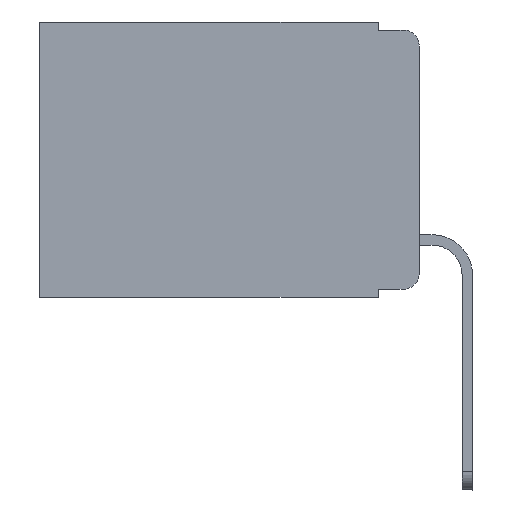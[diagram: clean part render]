
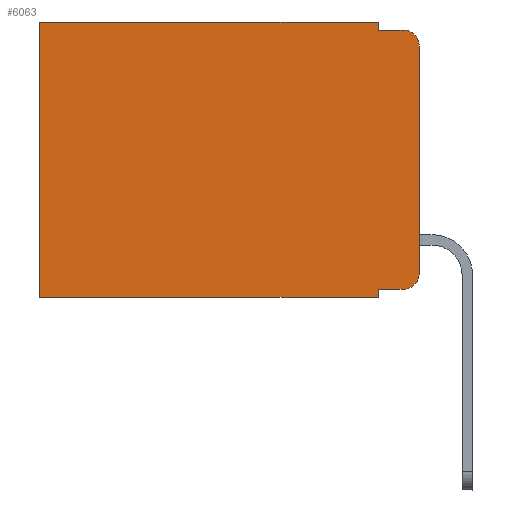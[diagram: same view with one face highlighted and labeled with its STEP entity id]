
A CAD part, left-side view. The second image highlights one B-rep face of the part: STEP entity #6063.
In plain terms, the highlighted planar face has unit normal (-1, 0, 0).
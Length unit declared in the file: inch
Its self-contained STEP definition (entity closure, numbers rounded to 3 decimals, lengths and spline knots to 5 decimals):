
#758 = CARTESIAN_POINT ( 'NONE',  ( 0.298, 0.473, -0.343 ) ) ;
#1137 = CARTESIAN_POINT ( 'NONE',  ( 0.298, 0., -0.03 ) ) ;
#1719 = VECTOR ( 'NONE', #22870, 39.37008 ) ;
#1736 = VERTEX_POINT ( 'NONE', #13730 ) ;
#1997 = CARTESIAN_POINT ( 'NONE',  ( 0.298, 0.02, -0.333 ) ) ;
#2095 = VERTEX_POINT ( 'NONE', #14075 ) ;
#2382 = VERTEX_POINT ( 'NONE', #1997 ) ;
#2701 = VECTOR ( 'NONE', #21764, 39.37008 ) ;
#2813 = VECTOR ( 'NONE', #3290, 39.37008 ) ;
#3217 = FACE_OUTER_BOUND ( 'NONE', #20248, .T. ) ;
#3290 = DIRECTION ( 'NONE',  ( 0., -1., 0. ) ) ;
#3627 = EDGE_CURVE ( 'NONE', #8540, #12872, #12313, .T. ) ;
#3735 = ORIENTED_EDGE ( 'NONE', *, *, #16666, .F. ) ;
#4019 = ORIENTED_EDGE ( 'NONE', *, *, #6465, .T. ) ;
#4311 = CARTESIAN_POINT ( 'NONE',  ( 0.298, 0.473, 0. ) ) ;
#5211 = CARTESIAN_POINT ( 'NONE',  ( 0.298, 0.051, 0. ) ) ;
#5522 = DIRECTION ( 'NONE',  ( -1., 0., 0. ) ) ;
#5570 = VECTOR ( 'NONE', #5739, 39.37008 ) ;
#5739 = DIRECTION ( 'NONE',  ( 0., 0., -1. ) ) ;
#5753 = EDGE_CURVE ( 'NONE', #10572, #1736, #19319, .T. ) ;
#5937 = LINE ( 'NONE', #4311, #19366 ) ;
#6043 = VERTEX_POINT ( 'NONE', #16541 ) ;
#6063 = ADVANCED_FACE ( 'NONE', ( #3217 ), #10880, .F. ) ;
#6457 = LINE ( 'NONE', #14120, #9599 ) ;
#6465 = EDGE_CURVE ( 'NONE', #23102, #6043, #6457, .T. ) ;
#6585 = CARTESIAN_POINT ( 'NONE',  ( 0.298, 0.02, -0.01 ) ) ;
#6776 = ORIENTED_EDGE ( 'NONE', *, *, #22594, .F. ) ;
#6887 = LINE ( 'NONE', #16563, #18034 ) ;
#7557 = LINE ( 'NONE', #15215, #1719 ) ;
#7729 = ORIENTED_EDGE ( 'NONE', *, *, #10859, .T. ) ;
#8098 = VECTOR ( 'NONE', #14165, 39.37008 ) ;
#8257 = EDGE_CURVE ( 'NONE', #10572, #2382, #10699, .T. ) ;
#8394 = ORIENTED_EDGE ( 'NONE', *, *, #5753, .F. ) ;
#8540 = VERTEX_POINT ( 'NONE', #1137 ) ;
#9599 = VECTOR ( 'NONE', #18025, 39.37008 ) ;
#9697 = VERTEX_POINT ( 'NONE', #10588 ) ;
#9969 = EDGE_CURVE ( 'NONE', #1736, #14996, #7557, .T. ) ;
#10539 = ORIENTED_EDGE ( 'NONE', *, *, #9969, .F. ) ;
#10572 = VERTEX_POINT ( 'NONE', #14507 ) ;
#10588 = CARTESIAN_POINT ( 'NONE',  ( 0.298, 0., -0.313 ) ) ;
#10699 = LINE ( 'NONE', #12584, #2813 ) ;
#10859 = EDGE_CURVE ( 'NONE', #6043, #14996, #5937, .T. ) ;
#10880 = PLANE ( 'NONE',  #16831 ) ;
#11693 = ORIENTED_EDGE ( 'NONE', *, *, #18721, .F. ) ;
#12313 = CIRCLE ( 'NONE', #21136, 0.02 ) ;
#12584 = CARTESIAN_POINT ( 'NONE',  ( 0.298, 0.051, -0.333 ) ) ;
#12769 = ORIENTED_EDGE ( 'NONE', *, *, #3627, .T. ) ;
#12872 = VERTEX_POINT ( 'NONE', #6585 ) ;
#13016 = CARTESIAN_POINT ( 'NONE',  ( 0.298, 0., 0. ) ) ;
#13553 = CARTESIAN_POINT ( 'NONE',  ( 0.298, 0.02, -0.03 ) ) ;
#13691 = AXIS2_PLACEMENT_3D ( 'NONE', #19484, #23235, #17346 ) ;
#13730 = CARTESIAN_POINT ( 'NONE',  ( 0.298, 0.051, -0.343 ) ) ;
#14075 = CARTESIAN_POINT ( 'NONE',  ( 0.298, 0.051, -0.01 ) ) ;
#14120 = CARTESIAN_POINT ( 'NONE',  ( 0.298, 0., 0. ) ) ;
#14165 = DIRECTION ( 'NONE',  ( 0., 0., -1. ) ) ;
#14507 = CARTESIAN_POINT ( 'NONE',  ( 0.298, 0.051, -0.333 ) ) ;
#14996 = VERTEX_POINT ( 'NONE', #758 ) ;
#15198 = DIRECTION ( 'NONE',  ( 0., 0., -1. ) ) ;
#15215 = CARTESIAN_POINT ( 'NONE',  ( 0.298, 0., -0.343 ) ) ;
#16541 = CARTESIAN_POINT ( 'NONE',  ( 0.298, 0.473, 0. ) ) ;
#16563 = CARTESIAN_POINT ( 'NONE',  ( 0.298, 0.051, -0.01 ) ) ;
#16666 = EDGE_CURVE ( 'NONE', #23102, #2095, #23268, .T. ) ;
#16831 = AXIS2_PLACEMENT_3D ( 'NONE', #13016, #18549, #20676 ) ;
#17346 = DIRECTION ( 'NONE',  ( 0., 0., -1. ) ) ;
#17428 = CARTESIAN_POINT ( 'NONE',  ( 0.298, 0.051, 0. ) ) ;
#17501 = CARTESIAN_POINT ( 'NONE',  ( 0.298, 0.051, 0. ) ) ;
#18025 = DIRECTION ( 'NONE',  ( 0., 1., 0. ) ) ;
#18034 = VECTOR ( 'NONE', #19961, 39.37008 ) ;
#18549 = DIRECTION ( 'NONE',  ( 1., 0., 0. ) ) ;
#18721 = EDGE_CURVE ( 'NONE', #2095, #12872, #6887, .T. ) ;
#18876 = ORIENTED_EDGE ( 'NONE', *, *, #20704, .T. ) ;
#19173 = ORIENTED_EDGE ( 'NONE', *, *, #8257, .T. ) ;
#19319 = LINE ( 'NONE', #17428, #5570 ) ;
#19340 = CIRCLE ( 'NONE', #13691, 0.02 ) ;
#19366 = VECTOR ( 'NONE', #23147, 39.37008 ) ;
#19484 = CARTESIAN_POINT ( 'NONE',  ( 0.298, 0.02, -0.313 ) ) ;
#19961 = DIRECTION ( 'NONE',  ( 0., -1., 0. ) ) ;
#20248 = EDGE_LOOP ( 'NONE', ( #6776, #12769, #11693, #3735, #4019, #7729, #10539, #8394, #19173, #18876 ) ) ;
#20676 = DIRECTION ( 'NONE',  ( 0., 0., -1. ) ) ;
#20704 = EDGE_CURVE ( 'NONE', #2382, #9697, #19340, .T. ) ;
#21136 = AXIS2_PLACEMENT_3D ( 'NONE', #13553, #5522, #15198 ) ;
#21764 = DIRECTION ( 'NONE',  ( 0., 0., -1. ) ) ;
#21829 = CARTESIAN_POINT ( 'NONE',  ( 0.298, 0., 0. ) ) ;
#22594 = EDGE_CURVE ( 'NONE', #8540, #9697, #23839, .T. ) ;
#22870 = DIRECTION ( 'NONE',  ( 0., 1., 0. ) ) ;
#23102 = VERTEX_POINT ( 'NONE', #5211 ) ;
#23147 = DIRECTION ( 'NONE',  ( 0., 0., -1. ) ) ;
#23235 = DIRECTION ( 'NONE',  ( -1., 0., 0. ) ) ;
#23268 = LINE ( 'NONE', #17501, #2701 ) ;
#23839 = LINE ( 'NONE', #21829, #8098 ) ;
